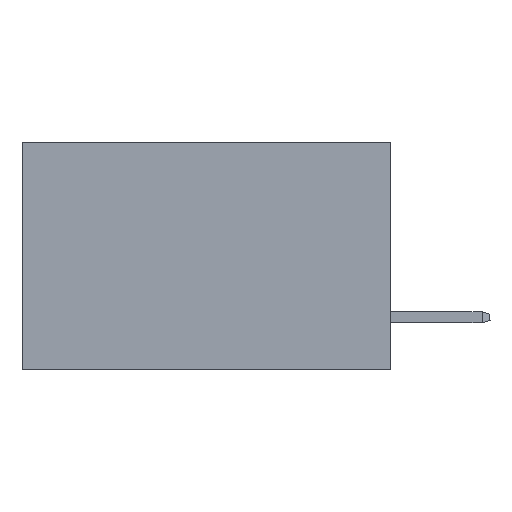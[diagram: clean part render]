
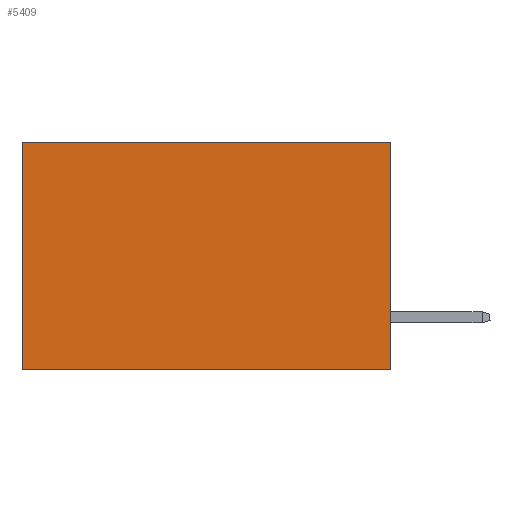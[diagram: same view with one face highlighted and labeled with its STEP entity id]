
A CAD part, left-side view. The second image highlights one B-rep face of the part: STEP entity #5409.
In plain terms, the highlighted planar face has unit normal (-1, 0, 0).
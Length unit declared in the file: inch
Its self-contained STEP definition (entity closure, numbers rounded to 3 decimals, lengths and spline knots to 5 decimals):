
#4617 = CARTESIAN_POINT ( 'NONE',  ( 0.2875, 0.6, -0.37 ) ) ;
#5409 = ADVANCED_FACE ( 'NONE', ( #30530 ), #36187, .F. ) ;
#5428 = EDGE_CURVE ( 'NONE', #34850, #23085, #8607, .T. ) ;
#5834 = VECTOR ( 'NONE', #15287, 39.37008 ) ;
#7254 = CARTESIAN_POINT ( 'NONE',  ( 0.2875, 0., 0. ) ) ;
#8607 = LINE ( 'NONE', #32648, #34910 ) ;
#8850 = ORIENTED_EDGE ( 'NONE', *, *, #19787, .F. ) ;
#10122 = ORIENTED_EDGE ( 'NONE', *, *, #28101, .T. ) ;
#11021 = CARTESIAN_POINT ( 'NONE',  ( 0.2875, 0., 0. ) ) ;
#12499 = ORIENTED_EDGE ( 'NONE', *, *, #23642, .T. ) ;
#12835 = CARTESIAN_POINT ( 'NONE',  ( 0.2875, 0.6, 0. ) ) ;
#13737 = DIRECTION ( 'NONE',  ( 1., 0., 0. ) ) ;
#15287 = DIRECTION ( 'NONE',  ( 0., 0., -1. ) ) ;
#17224 = LINE ( 'NONE', #12835, #5834 ) ;
#18377 = DIRECTION ( 'NONE',  ( 0., 1., 0. ) ) ;
#18508 = LINE ( 'NONE', #34153, #35654 ) ;
#19373 = DIRECTION ( 'NONE',  ( 0., 0., -1. ) ) ;
#19787 = EDGE_CURVE ( 'NONE', #23085, #26376, #18508, .T. ) ;
#20044 = DIRECTION ( 'NONE',  ( 0., 1., 0. ) ) ;
#20434 = EDGE_LOOP ( 'NONE', ( #10122, #8850, #26884, #12499 ) ) ;
#23085 = VERTEX_POINT ( 'NONE', #23112 ) ;
#23112 = CARTESIAN_POINT ( 'NONE',  ( 0.2875, 0., -0.37 ) ) ;
#23137 = CARTESIAN_POINT ( 'NONE',  ( 0.2875, 0.6, 0. ) ) ;
#23642 = EDGE_CURVE ( 'NONE', #34850, #27693, #29795, .T. ) ;
#23806 = CARTESIAN_POINT ( 'NONE',  ( 0.2875, 0., 0. ) ) ;
#26376 = VERTEX_POINT ( 'NONE', #4617 ) ;
#26884 = ORIENTED_EDGE ( 'NONE', *, *, #5428, .F. ) ;
#27693 = VERTEX_POINT ( 'NONE', #23137 ) ;
#28101 = EDGE_CURVE ( 'NONE', #27693, #26376, #17224, .T. ) ;
#29795 = LINE ( 'NONE', #7254, #30223 ) ;
#30223 = VECTOR ( 'NONE', #18377, 39.37008 ) ;
#30530 = FACE_OUTER_BOUND ( 'NONE', #20434, .T. ) ;
#32648 = CARTESIAN_POINT ( 'NONE',  ( 0.2875, 0., 0. ) ) ;
#33446 = DIRECTION ( 'NONE',  ( 0., 0., -1. ) ) ;
#34153 = CARTESIAN_POINT ( 'NONE',  ( 0.2875, 0., -0.37 ) ) ;
#34261 = AXIS2_PLACEMENT_3D ( 'NONE', #11021, #13737, #33446 ) ;
#34850 = VERTEX_POINT ( 'NONE', #23806 ) ;
#34910 = VECTOR ( 'NONE', #19373, 39.37008 ) ;
#35654 = VECTOR ( 'NONE', #20044, 39.37008 ) ;
#36187 = PLANE ( 'NONE',  #34261 ) ;
